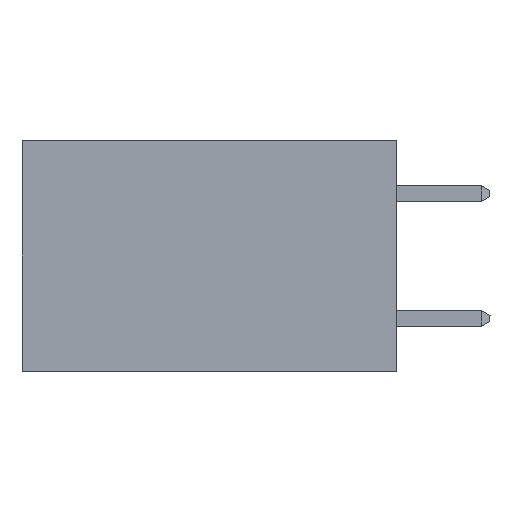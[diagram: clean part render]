
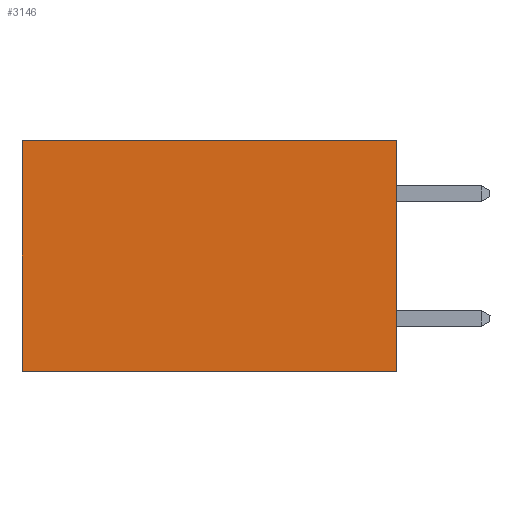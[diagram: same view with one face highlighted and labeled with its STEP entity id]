
A CAD part, left-side view. The second image highlights one B-rep face of the part: STEP entity #3146.
In plain terms, the highlighted planar face has unit normal (-1, 0, 0).
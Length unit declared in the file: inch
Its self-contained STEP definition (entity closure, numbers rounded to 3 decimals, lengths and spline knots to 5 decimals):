
#87 = ORIENTED_EDGE ( 'NONE', *, *, #236, .F. ) ;
#186 = EDGE_CURVE ( 'NONE', #10557, #8752, #818, .T. ) ;
#236 = EDGE_CURVE ( 'NONE', #8108, #3861, #8503, .T. ) ;
#818 = LINE ( 'NONE', #1209, #10769 ) ;
#982 = VECTOR ( 'NONE', #3100, 39.37008 ) ;
#1209 = CARTESIAN_POINT ( 'NONE',  ( 0.298, 0., 0. ) ) ;
#1426 = DIRECTION ( 'NONE',  ( 0., 0., -1. ) ) ;
#1431 = CARTESIAN_POINT ( 'NONE',  ( 0.298, 0.6, 0. ) ) ;
#2217 = ORIENTED_EDGE ( 'NONE', *, *, #10152, .T. ) ;
#2593 = ORIENTED_EDGE ( 'NONE', *, *, #6513, .F. ) ;
#2789 = PLANE ( 'NONE',  #8482 ) ;
#3100 = DIRECTION ( 'NONE',  ( 0., 1., 0. ) ) ;
#3146 = ADVANCED_FACE ( 'NONE', ( #11690 ), #2789, .F. ) ;
#3211 = VECTOR ( 'NONE', #8811, 39.37008 ) ;
#3418 = CARTESIAN_POINT ( 'NONE',  ( 0.298, 0.6, 0. ) ) ;
#3745 = CARTESIAN_POINT ( 'NONE',  ( 0.298, 0., 0. ) ) ;
#3861 = VERTEX_POINT ( 'NONE', #10222 ) ;
#4094 = CARTESIAN_POINT ( 'NONE',  ( 0.298, 0., -0.37 ) ) ;
#4381 = VECTOR ( 'NONE', #1426, 39.37008 ) ;
#5982 = DIRECTION ( 'NONE',  ( 0., 1., 0. ) ) ;
#6307 = CARTESIAN_POINT ( 'NONE',  ( 0.298, 0., 0. ) ) ;
#6410 = CARTESIAN_POINT ( 'NONE',  ( 0.298, 0., -0.37 ) ) ;
#6513 = EDGE_CURVE ( 'NONE', #10557, #8108, #8067, .T. ) ;
#7413 = ORIENTED_EDGE ( 'NONE', *, *, #186, .T. ) ;
#8067 = LINE ( 'NONE', #11044, #4381 ) ;
#8108 = VERTEX_POINT ( 'NONE', #6410 ) ;
#8482 = AXIS2_PLACEMENT_3D ( 'NONE', #3745, #10384, #11339 ) ;
#8503 = LINE ( 'NONE', #4094, #982 ) ;
#8752 = VERTEX_POINT ( 'NONE', #1431 ) ;
#8811 = DIRECTION ( 'NONE',  ( 0., 0., -1. ) ) ;
#10152 = EDGE_CURVE ( 'NONE', #8752, #3861, #12271, .T. ) ;
#10222 = CARTESIAN_POINT ( 'NONE',  ( 0.298, 0.6, -0.37 ) ) ;
#10384 = DIRECTION ( 'NONE',  ( 1., 0., 0. ) ) ;
#10418 = EDGE_LOOP ( 'NONE', ( #2217, #87, #2593, #7413 ) ) ;
#10557 = VERTEX_POINT ( 'NONE', #6307 ) ;
#10769 = VECTOR ( 'NONE', #5982, 39.37008 ) ;
#11044 = CARTESIAN_POINT ( 'NONE',  ( 0.298, 0., 0. ) ) ;
#11339 = DIRECTION ( 'NONE',  ( 0., 0., -1. ) ) ;
#11690 = FACE_OUTER_BOUND ( 'NONE', #10418, .T. ) ;
#12271 = LINE ( 'NONE', #3418, #3211 ) ;
